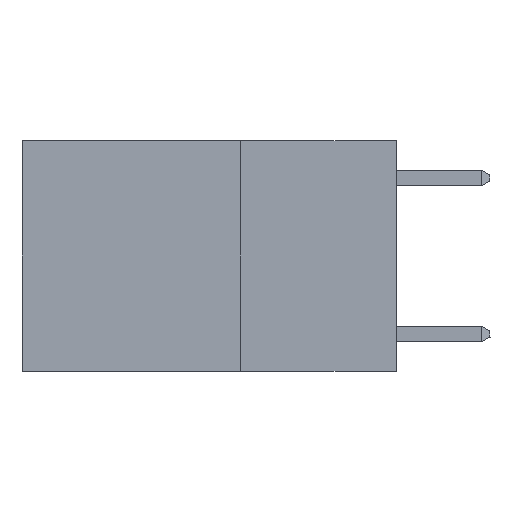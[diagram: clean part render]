
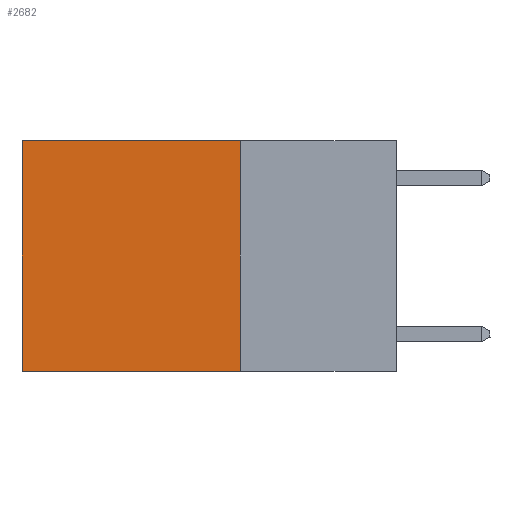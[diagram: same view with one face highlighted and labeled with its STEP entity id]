
A CAD part, left-side view. The second image highlights one B-rep face of the part: STEP entity #2682.
In plain terms, the highlighted planar face has unit normal (-1, 0, 0).
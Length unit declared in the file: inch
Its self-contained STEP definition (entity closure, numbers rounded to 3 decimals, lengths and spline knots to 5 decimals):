
#349 = CARTESIAN_POINT ( 'NONE',  ( 0.2625, 0.6, -0.37 ) ) ;
#1070 = FACE_OUTER_BOUND ( 'NONE', #4605, .T. ) ;
#1094 = DIRECTION ( 'NONE',  ( 0., 0., -1. ) ) ;
#1174 = VERTEX_POINT ( 'NONE', #6362 ) ;
#1252 = VECTOR ( 'NONE', #10719, 39.37008 ) ;
#1510 = EDGE_CURVE ( 'NONE', #1174, #10469, #6250, .T. ) ;
#2009 = CARTESIAN_POINT ( 'NONE',  ( 0.2625, 0.6, 0. ) ) ;
#2308 = CARTESIAN_POINT ( 'NONE',  ( 0.2625, 0.25, -0.37 ) ) ;
#2682 = ADVANCED_FACE ( 'NONE', ( #1070 ), #9515, .F. ) ;
#3261 = EDGE_CURVE ( 'NONE', #7082, #6686, #9576, .T. ) ;
#4513 = CARTESIAN_POINT ( 'NONE',  ( 0.2625, 0.6, 0. ) ) ;
#4595 = ORIENTED_EDGE ( 'NONE', *, *, #6770, .F. ) ;
#4605 = EDGE_LOOP ( 'NONE', ( #4633, #4595, #4800, #4774 ) ) ;
#4633 = ORIENTED_EDGE ( 'NONE', *, *, #3261, .T. ) ;
#4774 = ORIENTED_EDGE ( 'NONE', *, *, #9409, .T. ) ;
#4800 = ORIENTED_EDGE ( 'NONE', *, *, #1510, .F. ) ;
#5167 = DIRECTION ( 'NONE',  ( 0., 0., -1. ) ) ;
#5531 = CARTESIAN_POINT ( 'NONE',  ( 0.2625, 0.25, 0. ) ) ;
#5636 = AXIS2_PLACEMENT_3D ( 'NONE', #7797, #10386, #5167 ) ;
#5693 = LINE ( 'NONE', #2308, #9771 ) ;
#6138 = DIRECTION ( 'NONE',  ( 0., 1., 0. ) ) ;
#6250 = LINE ( 'NONE', #5531, #1252 ) ;
#6362 = CARTESIAN_POINT ( 'NONE',  ( 0.2625, 0.25, 0. ) ) ;
#6686 = VERTEX_POINT ( 'NONE', #349 ) ;
#6759 = VECTOR ( 'NONE', #6138, 39.37008 ) ;
#6770 = EDGE_CURVE ( 'NONE', #10469, #6686, #5693, .T. ) ;
#7082 = VERTEX_POINT ( 'NONE', #4513 ) ;
#7797 = CARTESIAN_POINT ( 'NONE',  ( 0.2625, 0.25, 0. ) ) ;
#7898 = CARTESIAN_POINT ( 'NONE',  ( 0.2625, 0.25, 0. ) ) ;
#9065 = VECTOR ( 'NONE', #1094, 39.37008 ) ;
#9068 = LINE ( 'NONE', #7898, #6759 ) ;
#9409 = EDGE_CURVE ( 'NONE', #1174, #7082, #9068, .T. ) ;
#9506 = DIRECTION ( 'NONE',  ( 0., 1., 0. ) ) ;
#9515 = PLANE ( 'NONE',  #5636 ) ;
#9576 = LINE ( 'NONE', #2009, #9065 ) ;
#9771 = VECTOR ( 'NONE', #9506, 39.37008 ) ;
#10386 = DIRECTION ( 'NONE',  ( 1., 0., 0. ) ) ;
#10469 = VERTEX_POINT ( 'NONE', #11218 ) ;
#10719 = DIRECTION ( 'NONE',  ( 0., 0., -1. ) ) ;
#11218 = CARTESIAN_POINT ( 'NONE',  ( 0.2625, 0.25, -0.37 ) ) ;
